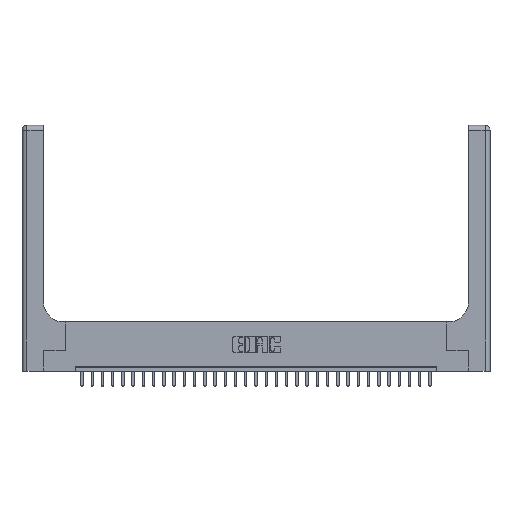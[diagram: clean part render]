
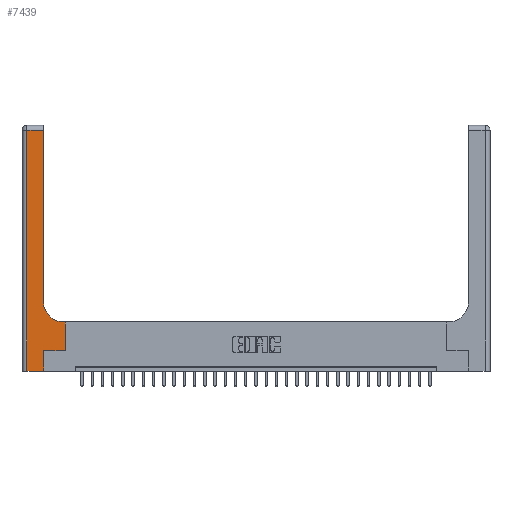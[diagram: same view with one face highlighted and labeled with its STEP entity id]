
A CAD part, top view. The second image highlights one B-rep face of the part: STEP entity #7439.
In plain terms, the highlighted planar face has unit normal (0, 0, 1).
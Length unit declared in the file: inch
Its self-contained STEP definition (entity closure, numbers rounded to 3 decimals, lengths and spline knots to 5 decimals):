
#158 = CARTESIAN_POINT ( 'NONE',  ( 0.265, 0., 0.37 ) ) ;
#854 = DIRECTION ( 'NONE',  ( -1., 0., 0. ) ) ;
#1217 = AXIS2_PLACEMENT_3D ( 'NONE', #7396, #27550, #854 ) ;
#1447 = LINE ( 'NONE', #9544, #18354 ) ;
#1584 = CARTESIAN_POINT ( 'NONE',  ( 0.26, 2.94, 0.37 ) ) ;
#2282 = EDGE_CURVE ( 'NONE', #8808, #21591, #3870, .T. ) ;
#2380 = ORIENTED_EDGE ( 'NONE', *, *, #26905, .T. ) ;
#2757 = ORIENTED_EDGE ( 'NONE', *, *, #12296, .T. ) ;
#3251 = ORIENTED_EDGE ( 'NONE', *, *, #16943, .T. ) ;
#3303 = DIRECTION ( 'NONE',  ( 0., 1., 0. ) ) ;
#3870 = LINE ( 'NONE', #3888, #11995 ) ;
#3888 = CARTESIAN_POINT ( 'NONE',  ( 0.26, 0.6, 0.37 ) ) ;
#3914 = VECTOR ( 'NONE', #3303, 39.37008 ) ;
#4366 = DIRECTION ( 'NONE',  ( 1., 0., 0. ) ) ;
#5111 = CARTESIAN_POINT ( 'NONE',  ( 0.265, 0.25, 0.37 ) ) ;
#5160 = DIRECTION ( 'NONE',  ( 1., 0., 0. ) ) ;
#5895 = DIRECTION ( 'NONE',  ( -1., 0., 0. ) ) ;
#6049 = DIRECTION ( 'NONE',  ( -1., 0., 0. ) ) ;
#6469 = EDGE_CURVE ( 'NONE', #16763, #27104, #12244, .T. ) ;
#6608 = LINE ( 'NONE', #9831, #3914 ) ;
#6783 = FACE_OUTER_BOUND ( 'NONE', #26497, .T. ) ;
#7396 = CARTESIAN_POINT ( 'NONE',  ( 0., 3., 0.37 ) ) ;
#7439 = ADVANCED_FACE ( 'NONE', ( #6783 ), #16070, .F. ) ;
#7481 = ORIENTED_EDGE ( 'NONE', *, *, #27825, .T. ) ;
#7660 = EDGE_CURVE ( 'NONE', #21591, #19208, #13170, .T. ) ;
#7877 = EDGE_CURVE ( 'NONE', #22705, #27759, #16877, .T. ) ;
#8294 = CARTESIAN_POINT ( 'NONE',  ( 0., 2.94, 0.37 ) ) ;
#8726 = DIRECTION ( 'NONE',  ( 0., 0., -1. ) ) ;
#8808 = VERTEX_POINT ( 'NONE', #14589 ) ;
#9302 = VERTEX_POINT ( 'NONE', #1584 ) ;
#9544 = CARTESIAN_POINT ( 'NONE',  ( 0., 0., 0.37 ) ) ;
#9588 = ORIENTED_EDGE ( 'NONE', *, *, #7877, .T. ) ;
#9641 = LINE ( 'NONE', #8294, #14989 ) ;
#9831 = CARTESIAN_POINT ( 'NONE',  ( 0.26, 3., 0.37 ) ) ;
#10386 = CARTESIAN_POINT ( 'NONE',  ( 0.06, 0., 0.37 ) ) ;
#10419 = CARTESIAN_POINT ( 'NONE',  ( 0.26, 0.85, 0.37 ) ) ;
#10501 = VECTOR ( 'NONE', #13421, 39.37008 ) ;
#11484 = ORIENTED_EDGE ( 'NONE', *, *, #2282, .T. ) ;
#11801 = EDGE_CURVE ( 'NONE', #9302, #16763, #9641, .T. ) ;
#11995 = VECTOR ( 'NONE', #6049, 39.37008 ) ;
#12244 = LINE ( 'NONE', #17732, #19998 ) ;
#12296 = EDGE_CURVE ( 'NONE', #27104, #19063, #1447, .T. ) ;
#12418 = CARTESIAN_POINT ( 'NONE',  ( 0.528, 0.25, 0.37 ) ) ;
#13170 = CIRCLE ( 'NONE', #20432, 0.25 ) ;
#13341 = VECTOR ( 'NONE', #23710, 39.37008 ) ;
#13421 = DIRECTION ( 'NONE',  ( 1., 0., 0. ) ) ;
#14589 = CARTESIAN_POINT ( 'NONE',  ( 0.528, 0.6, 0.37 ) ) ;
#14989 = VECTOR ( 'NONE', #5895, 39.37008 ) ;
#15635 = CARTESIAN_POINT ( 'NONE',  ( 0.51, 0.6, 0.37 ) ) ;
#15743 = DIRECTION ( 'NONE',  ( 0., -1., 0. ) ) ;
#16070 = PLANE ( 'NONE',  #1217 ) ;
#16427 = LINE ( 'NONE', #27378, #17113 ) ;
#16763 = VERTEX_POINT ( 'NONE', #18270 ) ;
#16877 = LINE ( 'NONE', #5111, #10501 ) ;
#16943 = EDGE_CURVE ( 'NONE', #27759, #8808, #16427, .T. ) ;
#17113 = VECTOR ( 'NONE', #23336, 39.37008 ) ;
#17732 = CARTESIAN_POINT ( 'NONE',  ( 0.06, 3., 0.37 ) ) ;
#17842 = CARTESIAN_POINT ( 'NONE',  ( 0.265, 0., 0.37 ) ) ;
#18270 = CARTESIAN_POINT ( 'NONE',  ( 0.06, 2.94, 0.37 ) ) ;
#18354 = VECTOR ( 'NONE', #5160, 39.37008 ) ;
#19063 = VERTEX_POINT ( 'NONE', #17842 ) ;
#19208 = VERTEX_POINT ( 'NONE', #10419 ) ;
#19456 = ORIENTED_EDGE ( 'NONE', *, *, #7660, .T. ) ;
#19998 = VECTOR ( 'NONE', #15743, 39.37008 ) ;
#20432 = AXIS2_PLACEMENT_3D ( 'NONE', #23894, #8726, #4366 ) ;
#20452 = ORIENTED_EDGE ( 'NONE', *, *, #11801, .T. ) ;
#21591 = VERTEX_POINT ( 'NONE', #15635 ) ;
#22705 = VERTEX_POINT ( 'NONE', #26049 ) ;
#23336 = DIRECTION ( 'NONE',  ( 0., 1., 0. ) ) ;
#23710 = DIRECTION ( 'NONE',  ( 0., 1., 0. ) ) ;
#23894 = CARTESIAN_POINT ( 'NONE',  ( 0.51, 0.85, 0.37 ) ) ;
#25369 = ORIENTED_EDGE ( 'NONE', *, *, #6469, .T. ) ;
#26049 = CARTESIAN_POINT ( 'NONE',  ( 0.265, 0.25, 0.37 ) ) ;
#26497 = EDGE_LOOP ( 'NONE', ( #2380, #20452, #25369, #2757, #7481, #9588, #3251, #11484, #19456 ) ) ;
#26905 = EDGE_CURVE ( 'NONE', #19208, #9302, #6608, .T. ) ;
#27104 = VERTEX_POINT ( 'NONE', #10386 ) ;
#27142 = LINE ( 'NONE', #158, #13341 ) ;
#27378 = CARTESIAN_POINT ( 'NONE',  ( 0.528, 0.25, 0.37 ) ) ;
#27550 = DIRECTION ( 'NONE',  ( 0., 0., -1. ) ) ;
#27759 = VERTEX_POINT ( 'NONE', #12418 ) ;
#27825 = EDGE_CURVE ( 'NONE', #19063, #22705, #27142, .T. ) ;
